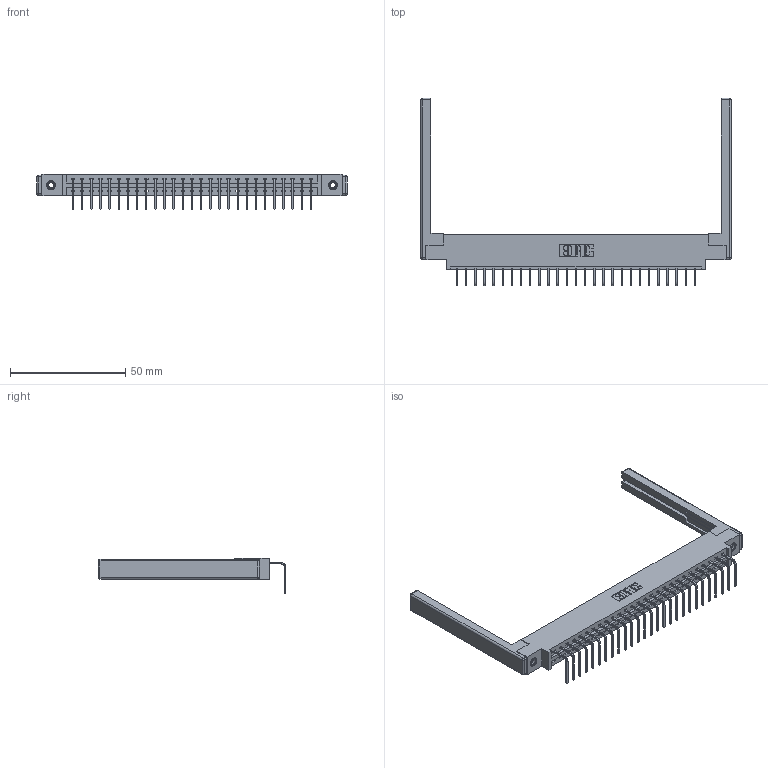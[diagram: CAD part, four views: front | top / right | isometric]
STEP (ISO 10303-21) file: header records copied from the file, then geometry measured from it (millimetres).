
FILE_DESCRIPTION (( 'STEP AP203' ), '1' );
FILE_NAME ('387-027-558-668.STEP', '2019-10-07T19:04:27', ( '' ), ( '' ), 'SwSTEP 2.0', 'SolidWorks 2016', '' );
FILE_SCHEMA (( 'CONFIG_CONTROL_DESIGN' ));
Length unit declared in the file: inch
Products named in the file (5): 345-292-001_558 Tail - 2; 307-220-068; 337 Part_0.170 Offset - 0.156 Dia-TI; 345-250-001_345-250-001-102; 387-027-558-668
Assembly tree (32 placements, depth 2):
  387-027-558-668
    337 Part_0.170 Offset - 0.156 Dia-TI
    345-292-001_558 Tail - 2  x27
    345-250-001_345-250-001-102  x2
    307-220-068  x2
Bounding box: 134.42 x 81.22 x 15.37 mm (x, y, z)
Volume: 18146.3 mm3; surface area: 18872.4 mm2
Topology: 32 solids, 32 shells, 2000 faces, 5951 edges, 3910 vertices
Faces by surface type: plane 1458, cylinder 518, cone 12, sphere 8, torus 4
Entity records: 24986 total; most frequent: CARTESIAN_POINT 4308, ORIENTED_EDGE 4260, DIRECTION 3730, EDGE_CURVE 2130, LINE 1952, VECTOR 1952, VERTEX_POINT 1410, AXIS2_PLACEMENT_3D 889
